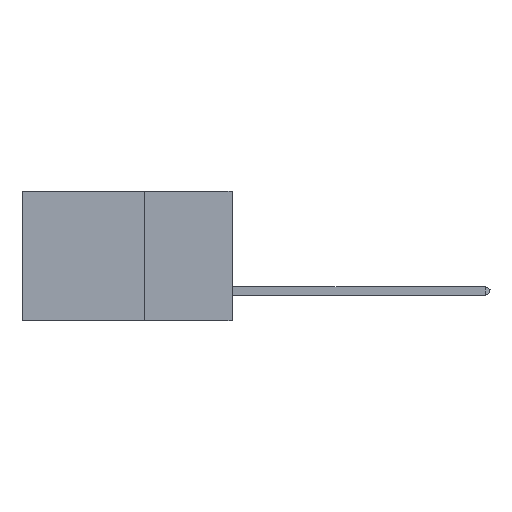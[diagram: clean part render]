
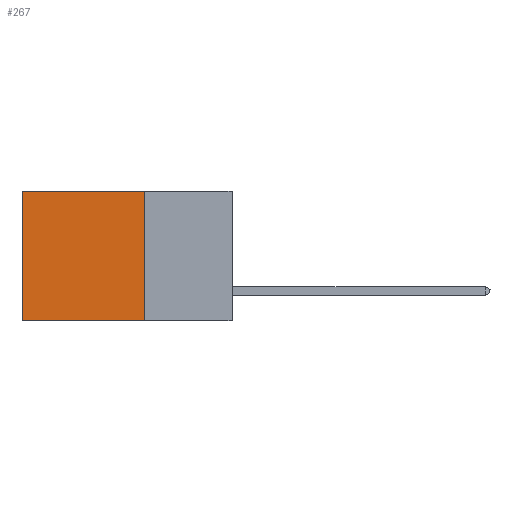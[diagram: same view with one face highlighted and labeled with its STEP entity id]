
A CAD part, left-side view. The second image highlights one B-rep face of the part: STEP entity #267.
In plain terms, the highlighted planar face has unit normal (-1, 0, 0).
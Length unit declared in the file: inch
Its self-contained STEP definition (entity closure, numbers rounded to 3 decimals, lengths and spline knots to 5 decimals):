
#267 = ADVANCED_FACE ( 'NONE', ( #6862 ), #18196, .F. ) ;
#365 = CARTESIAN_POINT ( 'NONE',  ( 0.2875, 0.25, 0. ) ) ;
#507 = LINE ( 'NONE', #7917, #2287 ) ;
#966 = ORIENTED_EDGE ( 'NONE', *, *, #18763, .T. ) ;
#1943 = CARTESIAN_POINT ( 'NONE',  ( 0.2875, 0.25, 0. ) ) ;
#2147 = VERTEX_POINT ( 'NONE', #15932 ) ;
#2287 = VECTOR ( 'NONE', #23350, 39.37008 ) ;
#4583 = DIRECTION ( 'NONE',  ( 0., 0., -1. ) ) ;
#4805 = DIRECTION ( 'NONE',  ( 0., 0., -1. ) ) ;
#4930 = EDGE_CURVE ( 'NONE', #23647, #5862, #507, .T. ) ;
#5862 = VERTEX_POINT ( 'NONE', #28412 ) ;
#6388 = CARTESIAN_POINT ( 'NONE',  ( 0.2875, 0.6, 0. ) ) ;
#6539 = CARTESIAN_POINT ( 'NONE',  ( 0.2875, 0.25, 0. ) ) ;
#6757 = EDGE_CURVE ( 'NONE', #10878, #23647, #12899, .T. ) ;
#6862 = FACE_OUTER_BOUND ( 'NONE', #15517, .T. ) ;
#7917 = CARTESIAN_POINT ( 'NONE',  ( 0.2875, 0.25, -0.37 ) ) ;
#8194 = ORIENTED_EDGE ( 'NONE', *, *, #19102, .T. ) ;
#10773 = DIRECTION ( 'NONE',  ( 0., 1., 0. ) ) ;
#10878 = VERTEX_POINT ( 'NONE', #6539 ) ;
#12899 = LINE ( 'NONE', #23608, #16714 ) ;
#13121 = ORIENTED_EDGE ( 'NONE', *, *, #4930, .F. ) ;
#15517 = EDGE_LOOP ( 'NONE', ( #966, #13121, #21916, #8194 ) ) ;
#15932 = CARTESIAN_POINT ( 'NONE',  ( 0.2875, 0.6, 0. ) ) ;
#16714 = VECTOR ( 'NONE', #21390, 39.37008 ) ;
#18196 = PLANE ( 'NONE',  #27812 ) ;
#18288 = LINE ( 'NONE', #6388, #27337 ) ;
#18763 = EDGE_CURVE ( 'NONE', #2147, #5862, #18288, .T. ) ;
#19102 = EDGE_CURVE ( 'NONE', #10878, #2147, #20361, .T. ) ;
#19440 = CARTESIAN_POINT ( 'NONE',  ( 0.2875, 0.25, -0.37 ) ) ;
#20361 = LINE ( 'NONE', #1943, #23484 ) ;
#20385 = DIRECTION ( 'NONE',  ( 1., 0., 0. ) ) ;
#21390 = DIRECTION ( 'NONE',  ( 0., 0., -1. ) ) ;
#21916 = ORIENTED_EDGE ( 'NONE', *, *, #6757, .F. ) ;
#23350 = DIRECTION ( 'NONE',  ( 0., 1., 0. ) ) ;
#23484 = VECTOR ( 'NONE', #10773, 39.37008 ) ;
#23608 = CARTESIAN_POINT ( 'NONE',  ( 0.2875, 0.25, 0. ) ) ;
#23647 = VERTEX_POINT ( 'NONE', #19440 ) ;
#27337 = VECTOR ( 'NONE', #4583, 39.37008 ) ;
#27812 = AXIS2_PLACEMENT_3D ( 'NONE', #365, #20385, #4805 ) ;
#28412 = CARTESIAN_POINT ( 'NONE',  ( 0.2875, 0.6, -0.37 ) ) ;
